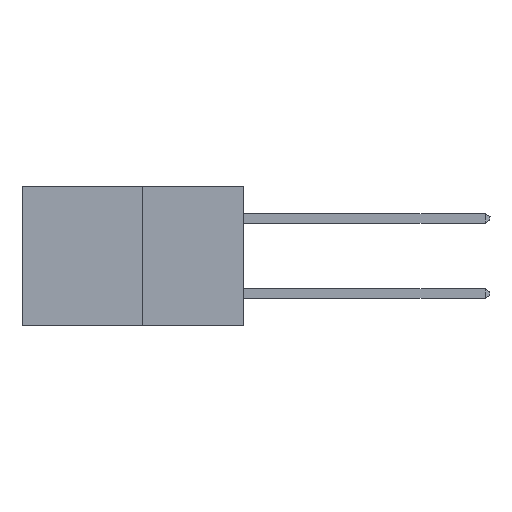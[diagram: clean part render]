
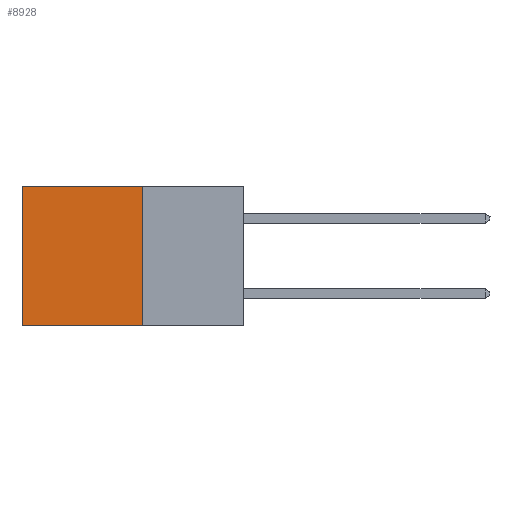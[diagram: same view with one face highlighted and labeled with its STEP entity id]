
A CAD part, left-side view. The second image highlights one B-rep face of the part: STEP entity #8928.
In plain terms, the highlighted planar face has unit normal (-1, 0, 0).
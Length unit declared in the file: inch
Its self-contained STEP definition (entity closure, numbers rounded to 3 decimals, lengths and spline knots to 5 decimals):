
#173 = LINE ( 'NONE', #8260, #11879 ) ;
#1151 = DIRECTION ( 'NONE',  ( 0., 1., 0. ) ) ;
#1414 = CARTESIAN_POINT ( 'NONE',  ( 0.277, 0.27, 0. ) ) ;
#1839 = ORIENTED_EDGE ( 'NONE', *, *, #6946, .F. ) ;
#2047 = CARTESIAN_POINT ( 'NONE',  ( 0.277, 0.59, 0. ) ) ;
#2565 = VERTEX_POINT ( 'NONE', #17474 ) ;
#2711 = EDGE_LOOP ( 'NONE', ( #11647, #5319, #1839, #5769 ) ) ;
#3289 = VECTOR ( 'NONE', #11103, 39.37008 ) ;
#3819 = EDGE_CURVE ( 'NONE', #16532, #2565, #173, .T. ) ;
#4696 = VERTEX_POINT ( 'NONE', #16113 ) ;
#5299 = PLANE ( 'NONE',  #15095 ) ;
#5319 = ORIENTED_EDGE ( 'NONE', *, *, #16671, .F. ) ;
#5769 = ORIENTED_EDGE ( 'NONE', *, *, #6182, .T. ) ;
#6182 = EDGE_CURVE ( 'NONE', #4696, #16532, #16097, .T. ) ;
#6301 = VECTOR ( 'NONE', #18173, 39.37008 ) ;
#6946 = EDGE_CURVE ( 'NONE', #4696, #11935, #17829, .T. ) ;
#8207 = CARTESIAN_POINT ( 'NONE',  ( 0.277, 0.27, -0.37 ) ) ;
#8209 = DIRECTION ( 'NONE',  ( 0., 0., -1. ) ) ;
#8217 = DIRECTION ( 'NONE',  ( 0., 0., -1. ) ) ;
#8260 = CARTESIAN_POINT ( 'NONE',  ( 0.277, 0.59, -0.37 ) ) ;
#8840 = VECTOR ( 'NONE', #1151, 39.37008 ) ;
#8928 = ADVANCED_FACE ( 'NONE', ( #11416 ), #5299, .F. ) ;
#10570 = LINE ( 'NONE', #8207, #3289 ) ;
#11103 = DIRECTION ( 'NONE',  ( 0., 1., 0. ) ) ;
#11416 = FACE_OUTER_BOUND ( 'NONE', #2711, .T. ) ;
#11647 = ORIENTED_EDGE ( 'NONE', *, *, #3819, .T. ) ;
#11879 = VECTOR ( 'NONE', #8217, 39.37008 ) ;
#11935 = VERTEX_POINT ( 'NONE', #18589 ) ;
#15095 = AXIS2_PLACEMENT_3D ( 'NONE', #15486, #16872, #8209 ) ;
#15486 = CARTESIAN_POINT ( 'NONE',  ( 0.277, 0.27, -0.37 ) ) ;
#16097 = LINE ( 'NONE', #1414, #8840 ) ;
#16113 = CARTESIAN_POINT ( 'NONE',  ( 0.277, 0.27, 0. ) ) ;
#16532 = VERTEX_POINT ( 'NONE', #2047 ) ;
#16671 = EDGE_CURVE ( 'NONE', #11935, #2565, #10570, .T. ) ;
#16872 = DIRECTION ( 'NONE',  ( 1., 0., 0. ) ) ;
#17474 = CARTESIAN_POINT ( 'NONE',  ( 0.277, 0.59, -0.37 ) ) ;
#17829 = LINE ( 'NONE', #17852, #6301 ) ;
#17852 = CARTESIAN_POINT ( 'NONE',  ( 0.277, 0.27, -0.37 ) ) ;
#18173 = DIRECTION ( 'NONE',  ( 0., 0., -1. ) ) ;
#18589 = CARTESIAN_POINT ( 'NONE',  ( 0.277, 0.27, -0.37 ) ) ;
